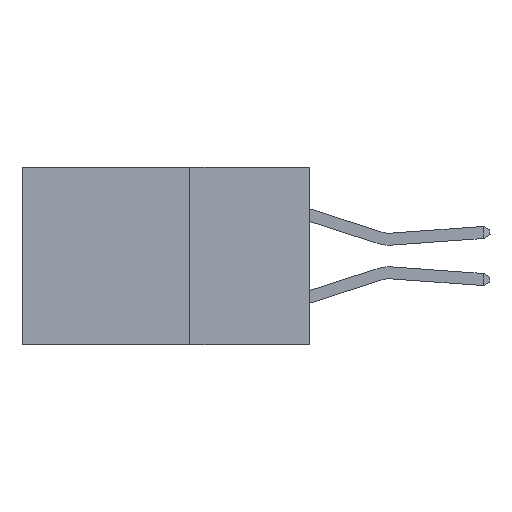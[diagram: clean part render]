
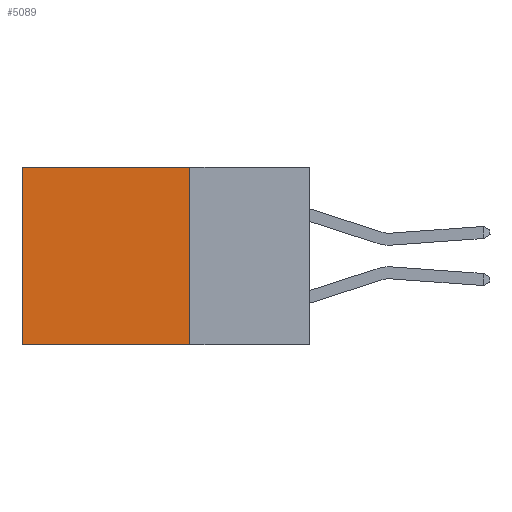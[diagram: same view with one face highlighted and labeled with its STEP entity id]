
A CAD part, left-side view. The second image highlights one B-rep face of the part: STEP entity #5089.
In plain terms, the highlighted planar face has unit normal (-1, 0, 0).
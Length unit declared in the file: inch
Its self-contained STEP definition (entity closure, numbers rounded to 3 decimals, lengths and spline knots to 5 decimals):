
#878 = CARTESIAN_POINT ( 'NONE',  ( 0.2615, 0.25, -0.37 ) ) ;
#980 = PLANE ( 'NONE',  #18679 ) ;
#1220 = ORIENTED_EDGE ( 'NONE', *, *, #15334, .F. ) ;
#1368 = ORIENTED_EDGE ( 'NONE', *, *, #2997, .F. ) ;
#1954 = CARTESIAN_POINT ( 'NONE',  ( 0.2615, 0.6, -0.37 ) ) ;
#2249 = LINE ( 'NONE', #1954, #9733 ) ;
#2513 = LINE ( 'NONE', #4079, #3590 ) ;
#2997 = EDGE_CURVE ( 'NONE', #20286, #18813, #4988, .T. ) ;
#3590 = VECTOR ( 'NONE', #16147, 39.37008 ) ;
#3982 = DIRECTION ( 'NONE',  ( 0., 0., -1. ) ) ;
#4079 = CARTESIAN_POINT ( 'NONE',  ( 0.2615, 0.25, 0. ) ) ;
#4933 = ORIENTED_EDGE ( 'NONE', *, *, #18766, .T. ) ;
#4988 = LINE ( 'NONE', #16292, #10533 ) ;
#5089 = ADVANCED_FACE ( 'NONE', ( #16834 ), #980, .F. ) ;
#5513 = VERTEX_POINT ( 'NONE', #9146 ) ;
#6705 = CARTESIAN_POINT ( 'NONE',  ( 0.2615, 0.25, 0. ) ) ;
#6827 = DIRECTION ( 'NONE',  ( 0., 0., -1. ) ) ;
#8427 = DIRECTION ( 'NONE',  ( 0., 0., -1. ) ) ;
#9146 = CARTESIAN_POINT ( 'NONE',  ( 0.2615, 0.6, 0. ) ) ;
#9363 = ORIENTED_EDGE ( 'NONE', *, *, #12234, .T. ) ;
#9733 = VECTOR ( 'NONE', #6827, 39.37008 ) ;
#10533 = VECTOR ( 'NONE', #8427, 39.37008 ) ;
#11184 = VECTOR ( 'NONE', #13351, 39.37008 ) ;
#11694 = CARTESIAN_POINT ( 'NONE',  ( 0.2615, 0.25, -0.37 ) ) ;
#12234 = EDGE_CURVE ( 'NONE', #5513, #16449, #2249, .T. ) ;
#12566 = CARTESIAN_POINT ( 'NONE',  ( 0.2615, 0.6, -0.37 ) ) ;
#13351 = DIRECTION ( 'NONE',  ( 0., 1., 0. ) ) ;
#15173 = DIRECTION ( 'NONE',  ( 1., 0., 0. ) ) ;
#15334 = EDGE_CURVE ( 'NONE', #18813, #16449, #17809, .T. ) ;
#16147 = DIRECTION ( 'NONE',  ( 0., 1., 0. ) ) ;
#16292 = CARTESIAN_POINT ( 'NONE',  ( 0.2615, 0.25, -0.37 ) ) ;
#16449 = VERTEX_POINT ( 'NONE', #12566 ) ;
#16834 = FACE_OUTER_BOUND ( 'NONE', #19133, .T. ) ;
#17809 = LINE ( 'NONE', #11694, #11184 ) ;
#18679 = AXIS2_PLACEMENT_3D ( 'NONE', #878, #15173, #3982 ) ;
#18766 = EDGE_CURVE ( 'NONE', #20286, #5513, #2513, .T. ) ;
#18813 = VERTEX_POINT ( 'NONE', #19557 ) ;
#19133 = EDGE_LOOP ( 'NONE', ( #9363, #1220, #1368, #4933 ) ) ;
#19557 = CARTESIAN_POINT ( 'NONE',  ( 0.2615, 0.25, -0.37 ) ) ;
#20286 = VERTEX_POINT ( 'NONE', #6705 ) ;
